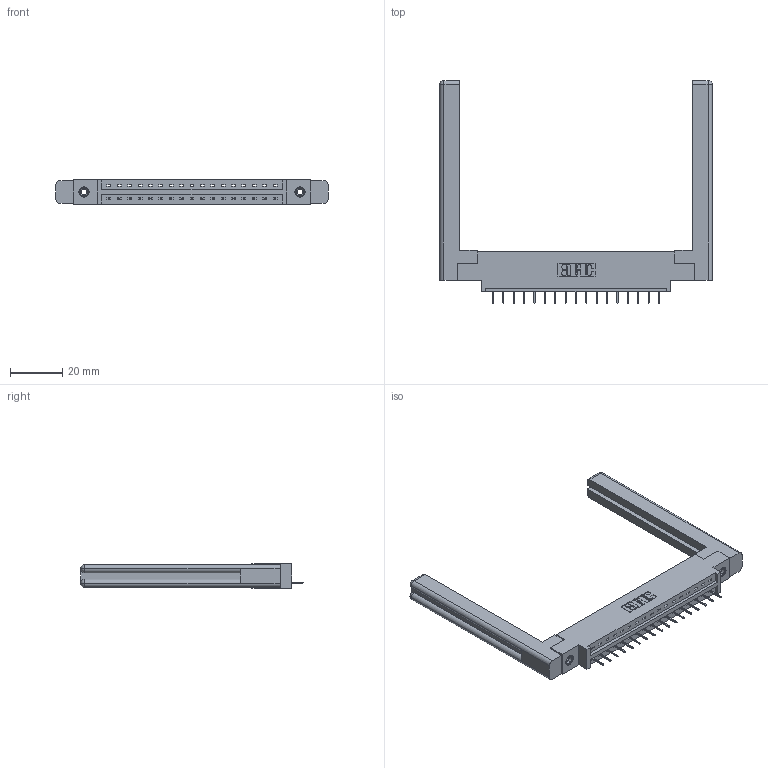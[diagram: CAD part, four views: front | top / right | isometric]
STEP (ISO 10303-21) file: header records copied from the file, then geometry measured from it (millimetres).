
FILE_DESCRIPTION (( 'STEP AP203' ), '1' );
FILE_NAME ('387-017-524-658.STEP', '2019-10-02T19:12:27', ( '' ), ( '' ), 'SwSTEP 2.0', 'SolidWorks 2016', '' );
FILE_SCHEMA (( 'CONFIG_CONTROL_DESIGN' ));
Length unit declared in the file: inch
Products named in the file (5): 387-017-524-658; 345-250-001_345-250-001-102; 307-220-058; 345-292-001_345-293-124; 337 Part_0.170 Offset - 0.156 Dia-TI
Assembly tree (22 placements, depth 2):
  387-017-524-658
    337 Part_0.170 Offset - 0.156 Dia-TI
    345-292-001_345-293-124  x17
    345-250-001_345-250-001-102  x2
    307-220-058  x2
Bounding box: 103.99 x 85.1 x 9.4 mm (x, y, z)
Volume: 17472.4 mm3; surface area: 15588.7 mm2
Topology: 22 solids, 22 shells, 1382 faces, 3941 edges, 2546 vertices
Faces by surface type: plane 1042, cylinder 316, cone 12, torus 12
Entity records: 18710 total; most frequent: CARTESIAN_POINT 3256, ORIENTED_EDGE 3148, DIRECTION 2812, EDGE_CURVE 1574, VECTOR 1402, LINE 1402, VERTEX_POINT 1038, AXIS2_PLACEMENT_3D 705
